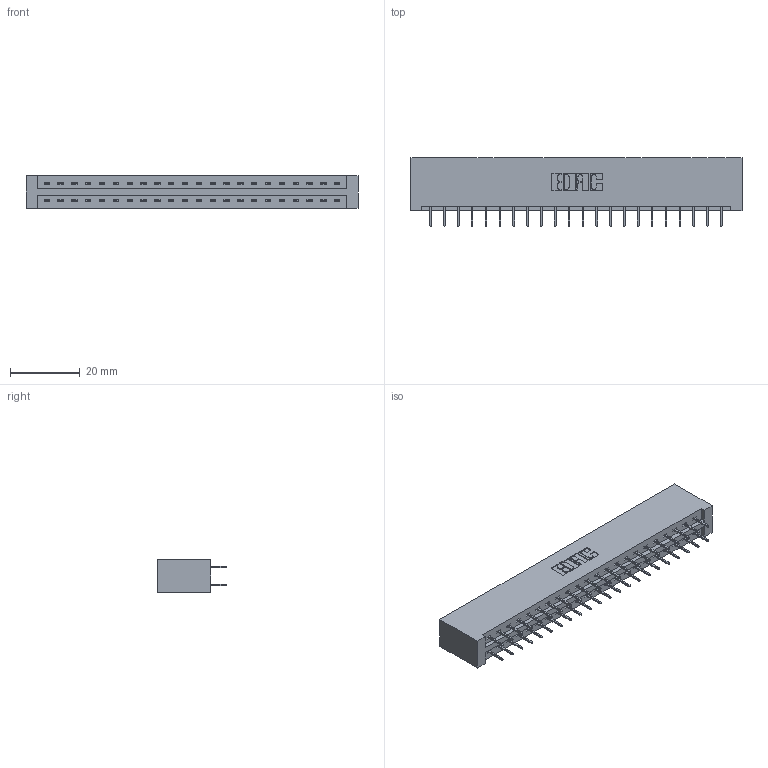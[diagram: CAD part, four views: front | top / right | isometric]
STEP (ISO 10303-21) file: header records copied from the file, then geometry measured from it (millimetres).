
FILE_DESCRIPTION (( 'STEP AP203' ), '1' );
FILE_NAME ('337-044-524-201.STEP', '2018-08-09T04:49:34', ( '' ), ( '' ), 'SwSTEP 2.0', 'SolidWorks 2016', '' );
FILE_SCHEMA (( 'CONFIG_CONTROL_DESIGN' ));
Length unit declared in the file: inch
Products named in the file (3): 337 Part_No Mounting Lugs; 345-292-001_345-293-124; 337-044-524-201
Assembly tree (45 placements, depth 2):
  337-044-524-201
    337 Part_No Mounting Lugs
    345-292-001_345-293-124  x44
Bounding box: 95.05 x 19.69 x 9.4 mm (x, y, z)
Volume: 10444.7 mm3; surface area: 11463.4 mm2
Topology: 45 solids, 45 shells, 2658 faces, 7547 edges, 4854 vertices
Faces by surface type: plane 2002, cylinder 656
Entity records: 19441 total; most frequent: CARTESIAN_POINT 3290, ORIENTED_EDGE 3226, DIRECTION 2829, EDGE_CURVE 1613, LINE 1497, VECTOR 1497, VERTEX_POINT 1070, AXIS2_PLACEMENT_3D 666
